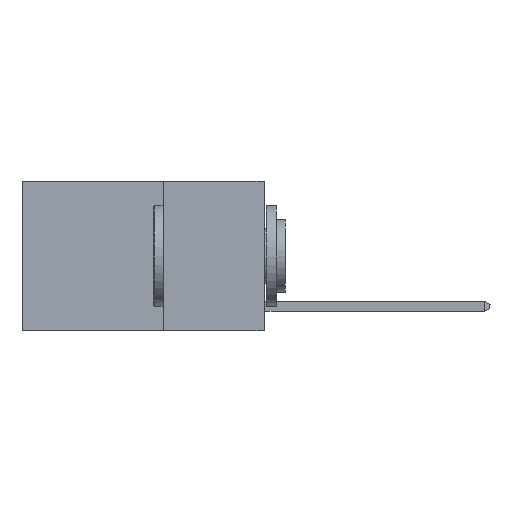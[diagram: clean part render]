
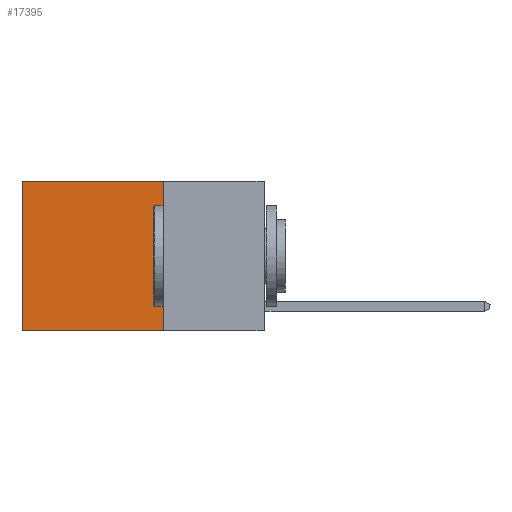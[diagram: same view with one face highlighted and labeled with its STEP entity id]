
A CAD part, left-side view. The second image highlights one B-rep face of the part: STEP entity #17395.
In plain terms, the highlighted planar face has unit normal (-1, 0, 0).
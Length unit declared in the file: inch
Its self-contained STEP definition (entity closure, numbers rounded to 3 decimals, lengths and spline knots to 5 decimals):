
#17 = DIRECTION ( 'NONE',  ( 0., 1., 0. ) ) ;
#192 = LINE ( 'NONE', #22275, #18867 ) ;
#383 = CARTESIAN_POINT ( 'NONE',  ( 0.2625, 0.25, 0. ) ) ;
#994 = ORIENTED_EDGE ( 'NONE', *, *, #10443, .T. ) ;
#1205 = AXIS2_PLACEMENT_3D ( 'NONE', #383, #4018, #16661 ) ;
#1897 = CARTESIAN_POINT ( 'NONE',  ( 0.2625, 0.6, 0. ) ) ;
#2469 = VERTEX_POINT ( 'NONE', #14866 ) ;
#3467 = VERTEX_POINT ( 'NONE', #10310 ) ;
#4018 = DIRECTION ( 'NONE',  ( 1., 0., 0. ) ) ;
#4023 = ORIENTED_EDGE ( 'NONE', *, *, #21656, .F. ) ;
#5329 = ORIENTED_EDGE ( 'NONE', *, *, #21924, .T. ) ;
#6097 = DIRECTION ( 'NONE',  ( 0., 1., 0. ) ) ;
#7918 = CARTESIAN_POINT ( 'NONE',  ( 0.2625, 0.25, 0. ) ) ;
#7982 = EDGE_LOOP ( 'NONE', ( #994, #4023, #19734, #5329 ) ) ;
#8537 = LINE ( 'NONE', #7918, #17597 ) ;
#8838 = VECTOR ( 'NONE', #17, 39.37008 ) ;
#9540 = VECTOR ( 'NONE', #15031, 39.37008 ) ;
#10310 = CARTESIAN_POINT ( 'NONE',  ( 0.2625, 0.6, -0.37 ) ) ;
#10443 = EDGE_CURVE ( 'NONE', #14911, #3467, #19158, .T. ) ;
#10659 = EDGE_CURVE ( 'NONE', #14913, #2469, #192, .T. ) ;
#13324 = DIRECTION ( 'NONE',  ( 0., 0., -1. ) ) ;
#14401 = CARTESIAN_POINT ( 'NONE',  ( 0.2625, 0.25, -0.37 ) ) ;
#14842 = PLANE ( 'NONE',  #1205 ) ;
#14866 = CARTESIAN_POINT ( 'NONE',  ( 0.2625, 0.25, -0.37 ) ) ;
#14911 = VERTEX_POINT ( 'NONE', #1897 ) ;
#14913 = VERTEX_POINT ( 'NONE', #18184 ) ;
#15031 = DIRECTION ( 'NONE',  ( 0., 0., -1. ) ) ;
#16661 = DIRECTION ( 'NONE',  ( 0., 0., -1. ) ) ;
#17395 = ADVANCED_FACE ( 'NONE', ( #22480 ), #14842, .F. ) ;
#17597 = VECTOR ( 'NONE', #6097, 39.37008 ) ;
#18080 = CARTESIAN_POINT ( 'NONE',  ( 0.2625, 0.6, 0. ) ) ;
#18184 = CARTESIAN_POINT ( 'NONE',  ( 0.2625, 0.25, 0. ) ) ;
#18867 = VECTOR ( 'NONE', #13324, 39.37008 ) ;
#19158 = LINE ( 'NONE', #18080, #9540 ) ;
#19572 = LINE ( 'NONE', #14401, #8838 ) ;
#19734 = ORIENTED_EDGE ( 'NONE', *, *, #10659, .F. ) ;
#21656 = EDGE_CURVE ( 'NONE', #2469, #3467, #19572, .T. ) ;
#21924 = EDGE_CURVE ( 'NONE', #14913, #14911, #8537, .T. ) ;
#22275 = CARTESIAN_POINT ( 'NONE',  ( 0.2625, 0.25, 0. ) ) ;
#22480 = FACE_OUTER_BOUND ( 'NONE', #7982, .T. ) ;
